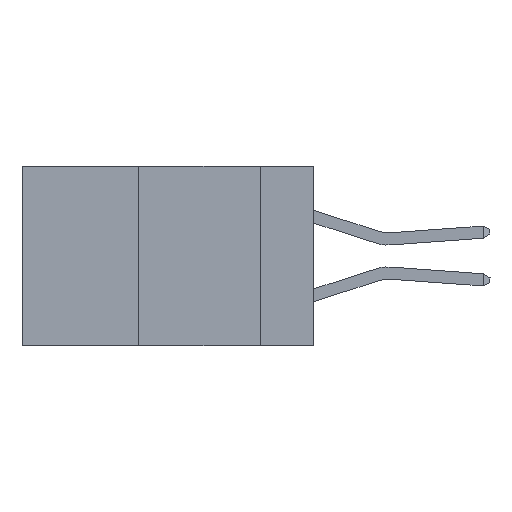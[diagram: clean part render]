
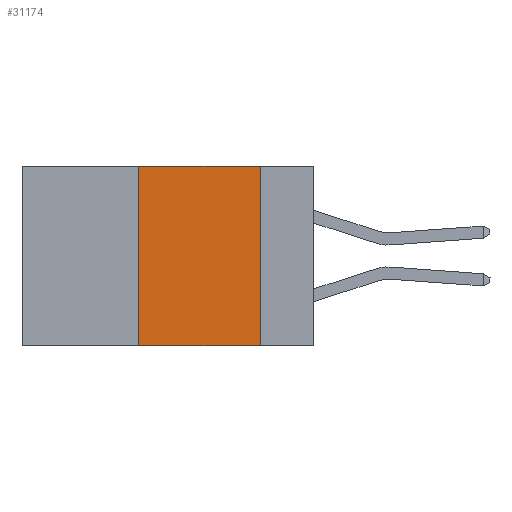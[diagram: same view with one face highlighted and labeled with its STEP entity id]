
A CAD part, left-side view. The second image highlights one B-rep face of the part: STEP entity #31174.
In plain terms, the highlighted planar face has unit normal (-1, 0, 0).
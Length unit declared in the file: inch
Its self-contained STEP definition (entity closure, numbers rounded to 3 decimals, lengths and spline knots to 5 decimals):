
#493 = CARTESIAN_POINT ( 'NONE',  ( 0., 0.36, 0. ) ) ;
#750 = LINE ( 'NONE', #11909, #33009 ) ;
#3988 = CARTESIAN_POINT ( 'NONE',  ( 0., 0.6, -0.37 ) ) ;
#5166 = ORIENTED_EDGE ( 'NONE', *, *, #27806, .F. ) ;
#5700 = FACE_OUTER_BOUND ( 'NONE', #34140, .T. ) ;
#5714 = DIRECTION ( 'NONE',  ( 0., 0., 1. ) ) ;
#7375 = VERTEX_POINT ( 'NONE', #27882 ) ;
#8287 = DIRECTION ( 'NONE',  ( 1., 0., 0. ) ) ;
#8844 = PLANE ( 'NONE',  #27304 ) ;
#9108 = DIRECTION ( 'NONE',  ( 0., -1., 0. ) ) ;
#11869 = VERTEX_POINT ( 'NONE', #12063 ) ;
#11909 = CARTESIAN_POINT ( 'NONE',  ( 0., 0.6, 0. ) ) ;
#11997 = LINE ( 'NONE', #3988, #23974 ) ;
#12063 = CARTESIAN_POINT ( 'NONE',  ( 0., 0.36, 0. ) ) ;
#16220 = ORIENTED_EDGE ( 'NONE', *, *, #22761, .F. ) ;
#17080 = CARTESIAN_POINT ( 'NONE',  ( 0., 0.6, 0. ) ) ;
#17743 = CARTESIAN_POINT ( 'NONE',  ( 0., 0.11, 0. ) ) ;
#18490 = DIRECTION ( 'NONE',  ( 0., 0., -1. ) ) ;
#20520 = ORIENTED_EDGE ( 'NONE', *, *, #25583, .T. ) ;
#21540 = VECTOR ( 'NONE', #18490, 39.37008 ) ;
#21970 = CARTESIAN_POINT ( 'NONE',  ( 0., 0.11, -0.37 ) ) ;
#22761 = EDGE_CURVE ( 'NONE', #32505, #23290, #29486, .T. ) ;
#23290 = VERTEX_POINT ( 'NONE', #21970 ) ;
#23974 = VECTOR ( 'NONE', #26751, 39.37008 ) ;
#25583 = EDGE_CURVE ( 'NONE', #7375, #23290, #11997, .T. ) ;
#26050 = LINE ( 'NONE', #493, #30692 ) ;
#26751 = DIRECTION ( 'NONE',  ( 0., -1., 0. ) ) ;
#27304 = AXIS2_PLACEMENT_3D ( 'NONE', #17080, #8287, #31066 ) ;
#27806 = EDGE_CURVE ( 'NONE', #11869, #32505, #750, .T. ) ;
#27882 = CARTESIAN_POINT ( 'NONE',  ( 0., 0.36, -0.37 ) ) ;
#29486 = LINE ( 'NONE', #17743, #21540 ) ;
#30692 = VECTOR ( 'NONE', #5714, 39.37008 ) ;
#31066 = DIRECTION ( 'NONE',  ( 0., 0., -1. ) ) ;
#31174 = ADVANCED_FACE ( 'NONE', ( #5700 ), #8844, .F. ) ;
#31895 = ORIENTED_EDGE ( 'NONE', *, *, #34116, .F. ) ;
#32505 = VERTEX_POINT ( 'NONE', #34849 ) ;
#33009 = VECTOR ( 'NONE', #9108, 39.37008 ) ;
#34116 = EDGE_CURVE ( 'NONE', #7375, #11869, #26050, .T. ) ;
#34140 = EDGE_LOOP ( 'NONE', ( #16220, #5166, #31895, #20520 ) ) ;
#34849 = CARTESIAN_POINT ( 'NONE',  ( 0., 0.11, 0. ) ) ;
